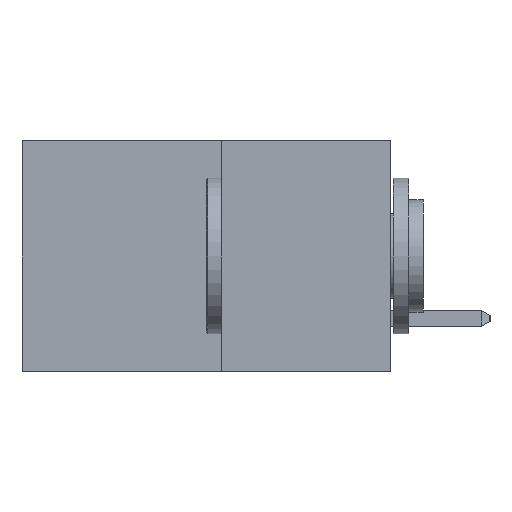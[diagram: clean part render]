
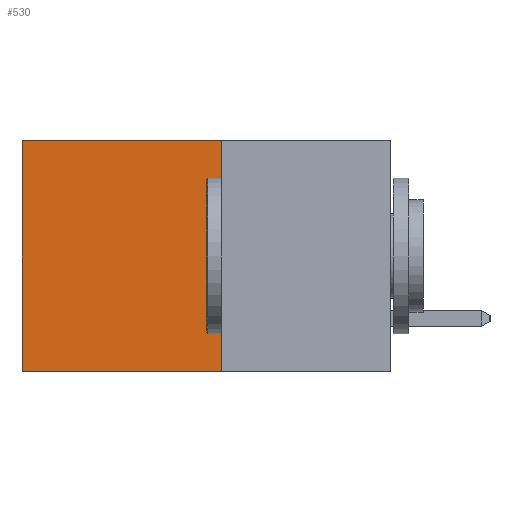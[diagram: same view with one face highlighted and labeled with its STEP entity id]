
A CAD part, left-side view. The second image highlights one B-rep face of the part: STEP entity #530.
In plain terms, the highlighted planar face has unit normal (-1, 0, 0).
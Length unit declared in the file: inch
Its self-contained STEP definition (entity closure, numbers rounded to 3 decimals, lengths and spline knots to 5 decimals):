
#202 = LINE ( 'NONE', #1618, #4654 ) ;
#353 = DIRECTION ( 'NONE',  ( 0., 0., -1. ) ) ;
#520 = DIRECTION ( 'NONE',  ( 0., 0., -1. ) ) ;
#530 = ADVANCED_FACE ( 'NONE', ( #1401 ), #6039, .F. ) ;
#1143 = DIRECTION ( 'NONE',  ( 1., 0., 0. ) ) ;
#1247 = CARTESIAN_POINT ( 'NONE',  ( 0.277, 0.27, -0.37 ) ) ;
#1401 = FACE_OUTER_BOUND ( 'NONE', #7045, .T. ) ;
#1536 = DIRECTION ( 'NONE',  ( 0., 1., 0. ) ) ;
#1618 = CARTESIAN_POINT ( 'NONE',  ( 0.277, 0.27, 0. ) ) ;
#1859 = EDGE_CURVE ( 'NONE', #6744, #7113, #8206, .T. ) ;
#2857 = CARTESIAN_POINT ( 'NONE',  ( 0.277, 0.59, 0. ) ) ;
#2971 = VERTEX_POINT ( 'NONE', #3579 ) ;
#3301 = ORIENTED_EDGE ( 'NONE', *, *, #4459, .F. ) ;
#3561 = ORIENTED_EDGE ( 'NONE', *, *, #5161, .T. ) ;
#3579 = CARTESIAN_POINT ( 'NONE',  ( 0.277, 0.59, -0.37 ) ) ;
#3623 = AXIS2_PLACEMENT_3D ( 'NONE', #1247, #1143, #353 ) ;
#4454 = CARTESIAN_POINT ( 'NONE',  ( 0.277, 0.59, -0.37 ) ) ;
#4459 = EDGE_CURVE ( 'NONE', #7113, #2971, #5955, .T. ) ;
#4654 = VECTOR ( 'NONE', #1536, 39.37008 ) ;
#5161 = EDGE_CURVE ( 'NONE', #6744, #9247, #202, .T. ) ;
#5955 = LINE ( 'NONE', #6321, #8140 ) ;
#6039 = PLANE ( 'NONE',  #3623 ) ;
#6321 = CARTESIAN_POINT ( 'NONE',  ( 0.277, 0.27, -0.37 ) ) ;
#6341 = DIRECTION ( 'NONE',  ( 0., 1., 0. ) ) ;
#6744 = VERTEX_POINT ( 'NONE', #8249 ) ;
#6903 = DIRECTION ( 'NONE',  ( 0., 0., -1. ) ) ;
#7045 = EDGE_LOOP ( 'NONE', ( #7193, #3301, #7733, #3561 ) ) ;
#7113 = VERTEX_POINT ( 'NONE', #7157 ) ;
#7157 = CARTESIAN_POINT ( 'NONE',  ( 0.277, 0.27, -0.37 ) ) ;
#7193 = ORIENTED_EDGE ( 'NONE', *, *, #8324, .T. ) ;
#7733 = ORIENTED_EDGE ( 'NONE', *, *, #1859, .F. ) ;
#8083 = CARTESIAN_POINT ( 'NONE',  ( 0.277, 0.27, -0.37 ) ) ;
#8140 = VECTOR ( 'NONE', #6341, 39.37008 ) ;
#8206 = LINE ( 'NONE', #8083, #10242 ) ;
#8249 = CARTESIAN_POINT ( 'NONE',  ( 0.277, 0.27, 0. ) ) ;
#8324 = EDGE_CURVE ( 'NONE', #9247, #2971, #10810, .T. ) ;
#8554 = VECTOR ( 'NONE', #6903, 39.37008 ) ;
#9247 = VERTEX_POINT ( 'NONE', #2857 ) ;
#10242 = VECTOR ( 'NONE', #520, 39.37008 ) ;
#10810 = LINE ( 'NONE', #4454, #8554 ) ;
